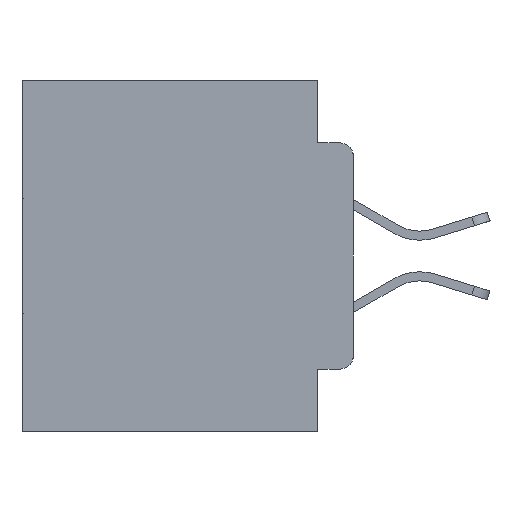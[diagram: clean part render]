
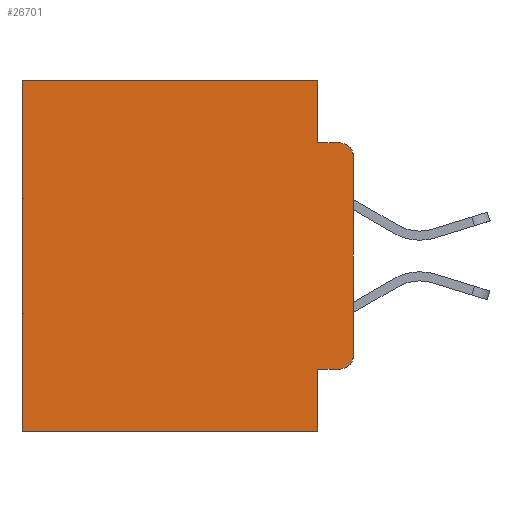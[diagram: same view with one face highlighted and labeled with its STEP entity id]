
A CAD part, left-side view. The second image highlights one B-rep face of the part: STEP entity #26701.
In plain terms, the highlighted planar face has unit normal (-1, 0, 0).
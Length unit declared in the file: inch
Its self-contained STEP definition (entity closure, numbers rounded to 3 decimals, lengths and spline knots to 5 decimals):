
#103 = EDGE_LOOP ( 'NONE', ( #10302, #28987, #16080, #2755, #15362, #13877, #15440, #9179, #15097, #7703 ) ) ;
#212 = EDGE_CURVE ( 'NONE', #20632, #16077, #5177, .T. ) ;
#1086 = DIRECTION ( 'NONE',  ( 0., 0., -1. ) ) ;
#1233 = VECTOR ( 'NONE', #30622, 39.37008 ) ;
#1928 = FACE_OUTER_BOUND ( 'NONE', #103, .T. ) ;
#1929 = EDGE_CURVE ( 'NONE', #16077, #10185, #27665, .T. ) ;
#2292 = CARTESIAN_POINT ( 'NONE',  ( 0.298, 0.051, -0.4115 ) ) ;
#2352 = CARTESIAN_POINT ( 'NONE',  ( 0.298, 0.051, 0. ) ) ;
#2755 = ORIENTED_EDGE ( 'NONE', *, *, #212, .F. ) ;
#2927 = CARTESIAN_POINT ( 'NONE',  ( 0.298, 0., -0.1085 ) ) ;
#4047 = AXIS2_PLACEMENT_3D ( 'NONE', #23313, #13962, #30290 ) ;
#4085 = VECTOR ( 'NONE', #12178, 39.37008 ) ;
#4467 = PLANE ( 'NONE',  #4047 ) ;
#5177 = LINE ( 'NONE', #2352, #16999 ) ;
#5188 = EDGE_CURVE ( 'NONE', #16566, #14152, #13562, .T. ) ;
#6795 = EDGE_CURVE ( 'NONE', #27189, #26413, #29924, .T. ) ;
#6938 = VERTEX_POINT ( 'NONE', #2927 ) ;
#7221 = CARTESIAN_POINT ( 'NONE',  ( 0.298, 0.473, 0. ) ) ;
#7666 = LINE ( 'NONE', #23666, #1233 ) ;
#7703 = ORIENTED_EDGE ( 'NONE', *, *, #8392, .T. ) ;
#8278 = CARTESIAN_POINT ( 'NONE',  ( 0.298, 0.02, -0.4115 ) ) ;
#8392 = EDGE_CURVE ( 'NONE', #11307, #30571, #12931, .T. ) ;
#8519 = DIRECTION ( 'NONE',  ( 0., 1., 0. ) ) ;
#8798 = CARTESIAN_POINT ( 'NONE',  ( 0.298, 0.051, 0. ) ) ;
#8834 = DIRECTION ( 'NONE',  ( 0., 0., -1. ) ) ;
#8990 = VECTOR ( 'NONE', #12360, 39.37008 ) ;
#9179 = ORIENTED_EDGE ( 'NONE', *, *, #5188, .F. ) ;
#9962 = EDGE_CURVE ( 'NONE', #16566, #11307, #7666, .T. ) ;
#10185 = VERTEX_POINT ( 'NONE', #22188 ) ;
#10302 = ORIENTED_EDGE ( 'NONE', *, *, #26260, .F. ) ;
#11307 = VERTEX_POINT ( 'NONE', #8278 ) ;
#11809 = CARTESIAN_POINT ( 'NONE',  ( 0.298, 0., -0.3915 ) ) ;
#12095 = VECTOR ( 'NONE', #8834, 39.37008 ) ;
#12178 = DIRECTION ( 'NONE',  ( 0., 1., 0. ) ) ;
#12360 = DIRECTION ( 'NONE',  ( 0., -1., 0. ) ) ;
#12931 = CIRCLE ( 'NONE', #21062, 0.02 ) ;
#13562 = LINE ( 'NONE', #8798, #12095 ) ;
#13869 = VECTOR ( 'NONE', #26501, 39.37008 ) ;
#13877 = ORIENTED_EDGE ( 'NONE', *, *, #6795, .T. ) ;
#13962 = DIRECTION ( 'NONE',  ( 1., 0., 0. ) ) ;
#14152 = VERTEX_POINT ( 'NONE', #29318 ) ;
#14338 = DIRECTION ( 'NONE',  ( -1., 0., 0. ) ) ;
#15097 = ORIENTED_EDGE ( 'NONE', *, *, #9962, .T. ) ;
#15362 = ORIENTED_EDGE ( 'NONE', *, *, #19932, .T. ) ;
#15380 = DIRECTION ( 'NONE',  ( -1., 0., 0. ) ) ;
#15440 = ORIENTED_EDGE ( 'NONE', *, *, #20546, .F. ) ;
#16077 = VERTEX_POINT ( 'NONE', #26817 ) ;
#16080 = ORIENTED_EDGE ( 'NONE', *, *, #1929, .F. ) ;
#16566 = VERTEX_POINT ( 'NONE', #2292 ) ;
#16670 = LINE ( 'NONE', #19131, #4085 ) ;
#16999 = VECTOR ( 'NONE', #20863, 39.37008 ) ;
#17752 = AXIS2_PLACEMENT_3D ( 'NONE', #28345, #14338, #29258 ) ;
#17853 = CARTESIAN_POINT ( 'NONE',  ( 0.298, 0., 0. ) ) ;
#18929 = DIRECTION ( 'NONE',  ( 0., 0., -1. ) ) ;
#19131 = CARTESIAN_POINT ( 'NONE',  ( 0.298, 0., -0.5 ) ) ;
#19922 = CARTESIAN_POINT ( 'NONE',  ( 0.298, 0.473, -0.5 ) ) ;
#19932 = EDGE_CURVE ( 'NONE', #20632, #27189, #27298, .T. ) ;
#20546 = EDGE_CURVE ( 'NONE', #14152, #26413, #16670, .T. ) ;
#20622 = CIRCLE ( 'NONE', #17752, 0.02 ) ;
#20632 = VERTEX_POINT ( 'NONE', #26635 ) ;
#20863 = DIRECTION ( 'NONE',  ( 0., 0., -1. ) ) ;
#21062 = AXIS2_PLACEMENT_3D ( 'NONE', #29356, #15380, #1086 ) ;
#21076 = VECTOR ( 'NONE', #8519, 39.37008 ) ;
#22188 = CARTESIAN_POINT ( 'NONE',  ( 0.298, 0.02, -0.0885 ) ) ;
#23313 = CARTESIAN_POINT ( 'NONE',  ( 0.298, 0., 0. ) ) ;
#23666 = CARTESIAN_POINT ( 'NONE',  ( 0.298, 0.051, -0.4115 ) ) ;
#24162 = CARTESIAN_POINT ( 'NONE',  ( 0.298, 0., 0. ) ) ;
#26260 = EDGE_CURVE ( 'NONE', #6938, #30571, #26345, .T. ) ;
#26345 = LINE ( 'NONE', #24162, #13869 ) ;
#26413 = VERTEX_POINT ( 'NONE', #19922 ) ;
#26501 = DIRECTION ( 'NONE',  ( 0., 0., -1. ) ) ;
#26635 = CARTESIAN_POINT ( 'NONE',  ( 0.298, 0.051, 0. ) ) ;
#26701 = ADVANCED_FACE ( 'NONE', ( #1928 ), #4467, .F. ) ;
#26817 = CARTESIAN_POINT ( 'NONE',  ( 0.298, 0.051, -0.0885 ) ) ;
#27189 = VERTEX_POINT ( 'NONE', #30270 ) ;
#27298 = LINE ( 'NONE', #17853, #21076 ) ;
#27665 = LINE ( 'NONE', #29916, #8990 ) ;
#28345 = CARTESIAN_POINT ( 'NONE',  ( 0.298, 0.02, -0.1085 ) ) ;
#28987 = ORIENTED_EDGE ( 'NONE', *, *, #29357, .T. ) ;
#29223 = VECTOR ( 'NONE', #18929, 39.37008 ) ;
#29258 = DIRECTION ( 'NONE',  ( 0., 0., -1. ) ) ;
#29318 = CARTESIAN_POINT ( 'NONE',  ( 0.298, 0.051, -0.5 ) ) ;
#29356 = CARTESIAN_POINT ( 'NONE',  ( 0.298, 0.02, -0.3915 ) ) ;
#29357 = EDGE_CURVE ( 'NONE', #6938, #10185, #20622, .T. ) ;
#29916 = CARTESIAN_POINT ( 'NONE',  ( 0.298, 0.051, -0.0885 ) ) ;
#29924 = LINE ( 'NONE', #7221, #29223 ) ;
#30270 = CARTESIAN_POINT ( 'NONE',  ( 0.298, 0.473, 0. ) ) ;
#30290 = DIRECTION ( 'NONE',  ( 0., 0., -1. ) ) ;
#30571 = VERTEX_POINT ( 'NONE', #11809 ) ;
#30622 = DIRECTION ( 'NONE',  ( 0., -1., 0. ) ) ;
